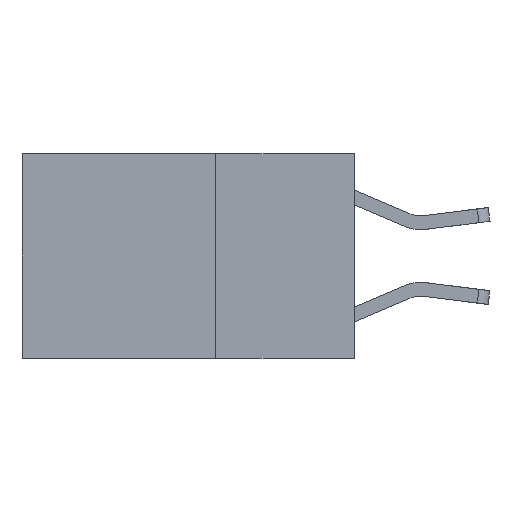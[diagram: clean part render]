
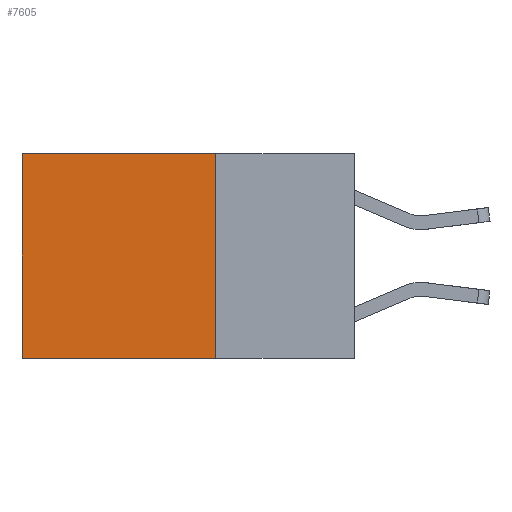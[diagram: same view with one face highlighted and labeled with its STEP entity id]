
A CAD part, left-side view. The second image highlights one B-rep face of the part: STEP entity #7605.
In plain terms, the highlighted planar face has unit normal (-1, 0, 0).
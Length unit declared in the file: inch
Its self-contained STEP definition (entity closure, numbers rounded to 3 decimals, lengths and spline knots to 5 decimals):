
#139 = CARTESIAN_POINT ( 'NONE',  ( 0.2625, 0.25, 0. ) ) ;
#487 = LINE ( 'NONE', #4025, #7384 ) ;
#742 = VECTOR ( 'NONE', #3517, 39.37008 ) ;
#849 = CARTESIAN_POINT ( 'NONE',  ( 0.2625, 0.25, -0.37 ) ) ;
#860 = VERTEX_POINT ( 'NONE', #2296 ) ;
#1263 = EDGE_CURVE ( 'NONE', #4960, #1560, #2271, .T. ) ;
#1560 = VERTEX_POINT ( 'NONE', #11120 ) ;
#2110 = DIRECTION ( 'NONE',  ( 0., 0., -1. ) ) ;
#2271 = LINE ( 'NONE', #849, #11879 ) ;
#2296 = CARTESIAN_POINT ( 'NONE',  ( 0.2625, 0.25, 0. ) ) ;
#2917 = ORIENTED_EDGE ( 'NONE', *, *, #1263, .F. ) ;
#3248 = LINE ( 'NONE', #7231, #742 ) ;
#3290 = LINE ( 'NONE', #139, #10407 ) ;
#3416 = CARTESIAN_POINT ( 'NONE',  ( 0.2625, 0.6, 0. ) ) ;
#3517 = DIRECTION ( 'NONE',  ( 0., 0., -1. ) ) ;
#3564 = AXIS2_PLACEMENT_3D ( 'NONE', #4277, #11711, #6176 ) ;
#4025 = CARTESIAN_POINT ( 'NONE',  ( 0.2625, 0.25, 0. ) ) ;
#4126 = ORIENTED_EDGE ( 'NONE', *, *, #7039, .T. ) ;
#4277 = CARTESIAN_POINT ( 'NONE',  ( 0.2625, 0.25, 0. ) ) ;
#4332 = FACE_OUTER_BOUND ( 'NONE', #10615, .T. ) ;
#4380 = EDGE_CURVE ( 'NONE', #8277, #1560, #3248, .T. ) ;
#4960 = VERTEX_POINT ( 'NONE', #6364 ) ;
#5787 = DIRECTION ( 'NONE',  ( 0., 1., 0. ) ) ;
#6176 = DIRECTION ( 'NONE',  ( 0., 0., -1. ) ) ;
#6364 = CARTESIAN_POINT ( 'NONE',  ( 0.2625, 0.25, -0.37 ) ) ;
#7039 = EDGE_CURVE ( 'NONE', #860, #8277, #3290, .T. ) ;
#7114 = EDGE_CURVE ( 'NONE', #860, #4960, #487, .T. ) ;
#7231 = CARTESIAN_POINT ( 'NONE',  ( 0.2625, 0.6, 0. ) ) ;
#7384 = VECTOR ( 'NONE', #2110, 39.37008 ) ;
#7605 = ADVANCED_FACE ( 'NONE', ( #4332 ), #10774, .F. ) ;
#7670 = DIRECTION ( 'NONE',  ( 0., 1., 0. ) ) ;
#8075 = ORIENTED_EDGE ( 'NONE', *, *, #7114, .F. ) ;
#8277 = VERTEX_POINT ( 'NONE', #3416 ) ;
#10320 = ORIENTED_EDGE ( 'NONE', *, *, #4380, .T. ) ;
#10407 = VECTOR ( 'NONE', #5787, 39.37008 ) ;
#10615 = EDGE_LOOP ( 'NONE', ( #10320, #2917, #8075, #4126 ) ) ;
#10774 = PLANE ( 'NONE',  #3564 ) ;
#11120 = CARTESIAN_POINT ( 'NONE',  ( 0.2625, 0.6, -0.37 ) ) ;
#11711 = DIRECTION ( 'NONE',  ( 1., 0., 0. ) ) ;
#11879 = VECTOR ( 'NONE', #7670, 39.37008 ) ;
